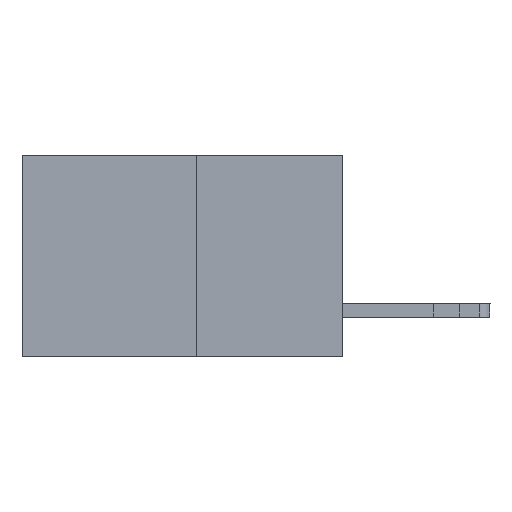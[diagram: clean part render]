
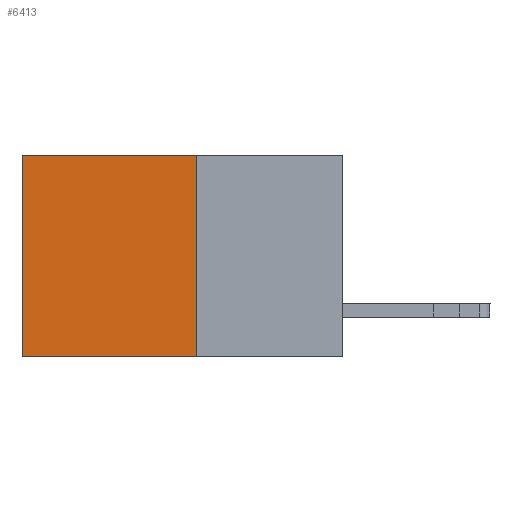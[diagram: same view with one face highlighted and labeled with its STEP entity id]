
A CAD part, left-side view. The second image highlights one B-rep face of the part: STEP entity #6413.
In plain terms, the highlighted planar face has unit normal (-1, 0, 0).
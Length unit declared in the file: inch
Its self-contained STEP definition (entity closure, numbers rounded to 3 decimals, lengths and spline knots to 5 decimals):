
#1810 = VECTOR ( 'NONE', #14666, 39.37008 ) ;
#2154 = VECTOR ( 'NONE', #10016, 39.37008 ) ;
#2191 = CARTESIAN_POINT ( 'NONE',  ( 0.277, 0.27, 0. ) ) ;
#2536 = CARTESIAN_POINT ( 'NONE',  ( 0.277, 0.59, -0.37 ) ) ;
#3401 = DIRECTION ( 'NONE',  ( 0., 1., 0. ) ) ;
#4165 = EDGE_CURVE ( 'NONE', #11786, #9694, #11557, .T. ) ;
#4706 = EDGE_CURVE ( 'NONE', #9694, #4978, #11727, .T. ) ;
#4978 = VERTEX_POINT ( 'NONE', #8850 ) ;
#5390 = VECTOR ( 'NONE', #3401, 39.37008 ) ;
#5414 = CARTESIAN_POINT ( 'NONE',  ( 0.277, 0.27, 0. ) ) ;
#5418 = CARTESIAN_POINT ( 'NONE',  ( 0.277, 0.27, -0.37 ) ) ;
#5439 = LINE ( 'NONE', #2536, #2154 ) ;
#5533 = ORIENTED_EDGE ( 'NONE', *, *, #9333, .T. ) ;
#6413 = ADVANCED_FACE ( 'NONE', ( #10146 ), #8257, .F. ) ;
#7628 = VERTEX_POINT ( 'NONE', #14895 ) ;
#8096 = DIRECTION ( 'NONE',  ( 1., 0., 0. ) ) ;
#8126 = DIRECTION ( 'NONE',  ( 0., 0., -1. ) ) ;
#8218 = CARTESIAN_POINT ( 'NONE',  ( 0.277, 0.27, -0.37 ) ) ;
#8257 = PLANE ( 'NONE',  #10369 ) ;
#8311 = VECTOR ( 'NONE', #12741, 39.37008 ) ;
#8850 = CARTESIAN_POINT ( 'NONE',  ( 0.277, 0.59, -0.37 ) ) ;
#9180 = ORIENTED_EDGE ( 'NONE', *, *, #4706, .F. ) ;
#9333 = EDGE_CURVE ( 'NONE', #11786, #7628, #11616, .T. ) ;
#9528 = ORIENTED_EDGE ( 'NONE', *, *, #14026, .T. ) ;
#9694 = VERTEX_POINT ( 'NONE', #5418 ) ;
#10016 = DIRECTION ( 'NONE',  ( 0., 0., -1. ) ) ;
#10146 = FACE_OUTER_BOUND ( 'NONE', #14144, .T. ) ;
#10369 = AXIS2_PLACEMENT_3D ( 'NONE', #8218, #8096, #8126 ) ;
#11557 = LINE ( 'NONE', #13200, #8311 ) ;
#11616 = LINE ( 'NONE', #2191, #5390 ) ;
#11727 = LINE ( 'NONE', #14628, #1810 ) ;
#11786 = VERTEX_POINT ( 'NONE', #5414 ) ;
#12128 = ORIENTED_EDGE ( 'NONE', *, *, #4165, .F. ) ;
#12741 = DIRECTION ( 'NONE',  ( 0., 0., -1. ) ) ;
#13200 = CARTESIAN_POINT ( 'NONE',  ( 0.277, 0.27, -0.37 ) ) ;
#14026 = EDGE_CURVE ( 'NONE', #7628, #4978, #5439, .T. ) ;
#14144 = EDGE_LOOP ( 'NONE', ( #9528, #9180, #12128, #5533 ) ) ;
#14628 = CARTESIAN_POINT ( 'NONE',  ( 0.277, 0.27, -0.37 ) ) ;
#14666 = DIRECTION ( 'NONE',  ( 0., 1., 0. ) ) ;
#14895 = CARTESIAN_POINT ( 'NONE',  ( 0.277, 0.59, 0. ) ) ;
